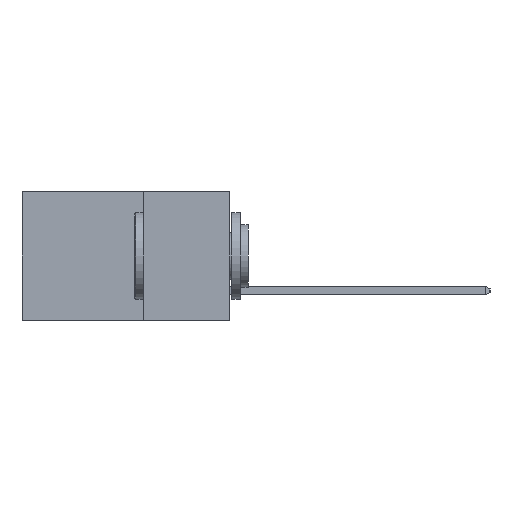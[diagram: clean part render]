
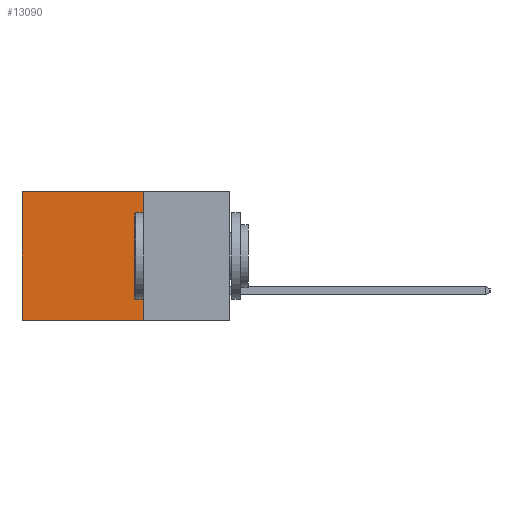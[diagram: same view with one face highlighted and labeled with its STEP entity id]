
A CAD part, left-side view. The second image highlights one B-rep face of the part: STEP entity #13090.
In plain terms, the highlighted planar face has unit normal (-1, 0, 0).
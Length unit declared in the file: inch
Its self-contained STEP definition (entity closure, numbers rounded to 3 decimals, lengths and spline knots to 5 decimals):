
#209 = ORIENTED_EDGE ( 'NONE', *, *, #12511, .F. ) ;
#273 = LINE ( 'NONE', #9397, #10943 ) ;
#499 = CARTESIAN_POINT ( 'NONE',  ( 0.298, 0.25, 0. ) ) ;
#773 = ORIENTED_EDGE ( 'NONE', *, *, #6010, .T. ) ;
#1411 = ORIENTED_EDGE ( 'NONE', *, *, #12980, .F. ) ;
#1747 = EDGE_CURVE ( 'NONE', #3554, #15180, #14321, .T. ) ;
#1807 = FACE_OUTER_BOUND ( 'NONE', #5966, .T. ) ;
#2722 = DIRECTION ( 'NONE',  ( 1., 0., 0. ) ) ;
#3057 = ORIENTED_EDGE ( 'NONE', *, *, #1747, .T. ) ;
#3117 = VECTOR ( 'NONE', #5789, 39.37008 ) ;
#3554 = VERTEX_POINT ( 'NONE', #5518 ) ;
#3724 = VERTEX_POINT ( 'NONE', #499 ) ;
#3914 = CARTESIAN_POINT ( 'NONE',  ( 0.298, 0.6, -0.37 ) ) ;
#4458 = VECTOR ( 'NONE', #9760, 39.37008 ) ;
#5518 = CARTESIAN_POINT ( 'NONE',  ( 0.298, 0.6, 0. ) ) ;
#5649 = CARTESIAN_POINT ( 'NONE',  ( 0.298, 0.25, 0. ) ) ;
#5789 = DIRECTION ( 'NONE',  ( 0., 1., 0. ) ) ;
#5966 = EDGE_LOOP ( 'NONE', ( #3057, #1411, #209, #773 ) ) ;
#6010 = EDGE_CURVE ( 'NONE', #3724, #3554, #14129, .T. ) ;
#6716 = DIRECTION ( 'NONE',  ( 0., 1., 0. ) ) ;
#6804 = CARTESIAN_POINT ( 'NONE',  ( 0.298, 0.25, -0.37 ) ) ;
#6896 = PLANE ( 'NONE',  #8943 ) ;
#7053 = VECTOR ( 'NONE', #11293, 39.37008 ) ;
#7638 = CARTESIAN_POINT ( 'NONE',  ( 0.298, 0.6, 0. ) ) ;
#8943 = AXIS2_PLACEMENT_3D ( 'NONE', #11020, #2722, #12409 ) ;
#9397 = CARTESIAN_POINT ( 'NONE',  ( 0.298, 0.25, -0.37 ) ) ;
#9760 = DIRECTION ( 'NONE',  ( 0., 0., -1. ) ) ;
#10943 = VECTOR ( 'NONE', #6716, 39.37008 ) ;
#11020 = CARTESIAN_POINT ( 'NONE',  ( 0.298, 0.25, 0. ) ) ;
#11293 = DIRECTION ( 'NONE',  ( 0., 0., -1. ) ) ;
#12409 = DIRECTION ( 'NONE',  ( 0., 0., -1. ) ) ;
#12511 = EDGE_CURVE ( 'NONE', #3724, #14224, #15401, .T. ) ;
#12980 = EDGE_CURVE ( 'NONE', #14224, #15180, #273, .T. ) ;
#13090 = ADVANCED_FACE ( 'NONE', ( #1807 ), #6896, .F. ) ;
#14129 = LINE ( 'NONE', #5649, #3117 ) ;
#14224 = VERTEX_POINT ( 'NONE', #6804 ) ;
#14321 = LINE ( 'NONE', #7638, #7053 ) ;
#15180 = VERTEX_POINT ( 'NONE', #3914 ) ;
#15401 = LINE ( 'NONE', #16545, #4458 ) ;
#16545 = CARTESIAN_POINT ( 'NONE',  ( 0.298, 0.25, 0. ) ) ;
